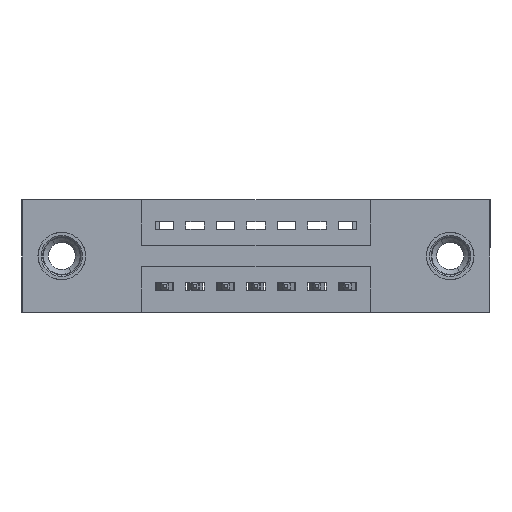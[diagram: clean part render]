
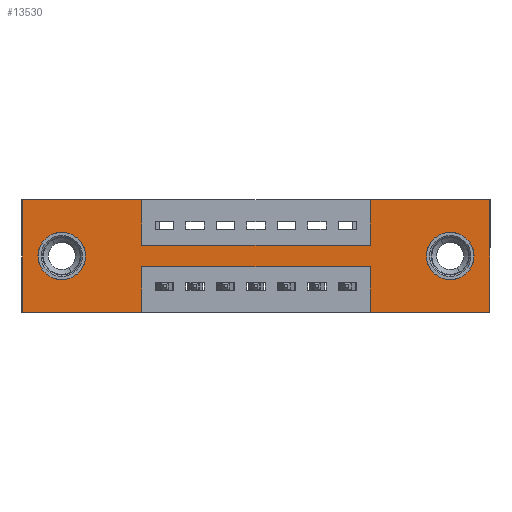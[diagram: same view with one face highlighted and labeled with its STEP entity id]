
A CAD part, front view. The second image highlights one B-rep face of the part: STEP entity #13530.
In plain terms, the highlighted planar face has unit normal (0, -1, 0).
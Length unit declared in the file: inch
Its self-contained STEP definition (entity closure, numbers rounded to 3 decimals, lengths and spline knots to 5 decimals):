
#209 = CIRCLE ( 'NONE', #303, 0.078 ) ;
#303 = AXIS2_PLACEMENT_3D ( 'NONE', #9126, #6802, #10121 ) ;
#385 = CARTESIAN_POINT ( 'NONE',  ( 0.3925, 0., -0.15 ) ) ;
#406 = VERTEX_POINT ( 'NONE', #3252 ) ;
#407 = VERTEX_POINT ( 'NONE', #1357 ) ;
#859 = DIRECTION ( 'NONE',  ( 1., 0., 0. ) ) ;
#923 = ORIENTED_EDGE ( 'NONE', *, *, #13395, .F. ) ;
#991 = EDGE_CURVE ( 'NONE', #10062, #406, #4878, .T. ) ;
#1077 = CIRCLE ( 'NONE', #7684, 0.078 ) ;
#1160 = LINE ( 'NONE', #14517, #9852 ) ;
#1196 = CARTESIAN_POINT ( 'NONE',  ( 1.1425, 0., -0.22 ) ) ;
#1280 = FACE_BOUND ( 'NONE', #7877, .T. ) ;
#1357 = CARTESIAN_POINT ( 'NONE',  ( 1.1425, 0., 0. ) ) ;
#1489 = LINE ( 'NONE', #6296, #6278 ) ;
#1538 = VERTEX_POINT ( 'NONE', #8342 ) ;
#1548 = ORIENTED_EDGE ( 'NONE', *, *, #2887, .F. ) ;
#1566 = ORIENTED_EDGE ( 'NONE', *, *, #13755, .F. ) ;
#1623 = CARTESIAN_POINT ( 'NONE',  ( 0., 0., -0.37 ) ) ;
#1640 = DIRECTION ( 'NONE',  ( 1., 0., 0. ) ) ;
#1660 = VERTEX_POINT ( 'NONE', #14369 ) ;
#1757 = CARTESIAN_POINT ( 'NONE',  ( 0.3925, 0., 0. ) ) ;
#1852 = ORIENTED_EDGE ( 'NONE', *, *, #10573, .F. ) ;
#1982 = PLANE ( 'NONE',  #3138 ) ;
#2019 = DIRECTION ( 'NONE',  ( 0., 0., 1. ) ) ;
#2030 = DIRECTION ( 'NONE',  ( 0., 0., 1. ) ) ;
#2088 = AXIS2_PLACEMENT_3D ( 'NONE', #5522, #3128, #4390 ) ;
#2141 = CARTESIAN_POINT ( 'NONE',  ( 0.13, 0., -0.107 ) ) ;
#2337 = ORIENTED_EDGE ( 'NONE', *, *, #12389, .F. ) ;
#2432 = DIRECTION ( 'NONE',  ( 0., 0., 1. ) ) ;
#2887 = EDGE_CURVE ( 'NONE', #8655, #12697, #8197, .T. ) ;
#3082 = EDGE_CURVE ( 'NONE', #406, #10062, #209, .T. ) ;
#3112 = CARTESIAN_POINT ( 'NONE',  ( 0., 0., -0.37 ) ) ;
#3128 = DIRECTION ( 'NONE',  ( 0., 1., 0. ) ) ;
#3138 = AXIS2_PLACEMENT_3D ( 'NONE', #3112, #5222, #14304 ) ;
#3252 = CARTESIAN_POINT ( 'NONE',  ( 1.405, 0., -0.107 ) ) ;
#3278 = VECTOR ( 'NONE', #859, 39.37008 ) ;
#3325 = ORIENTED_EDGE ( 'NONE', *, *, #3082, .T. ) ;
#3356 = CARTESIAN_POINT ( 'NONE',  ( 1.1425, 0., -0.37 ) ) ;
#3400 = LINE ( 'NONE', #11828, #4587 ) ;
#3623 = LINE ( 'NONE', #12787, #11231 ) ;
#3951 = DIRECTION ( 'NONE',  ( -1., 0., 0. ) ) ;
#3960 = CARTESIAN_POINT ( 'NONE',  ( 0.3925, 0., -0.37 ) ) ;
#3966 = CARTESIAN_POINT ( 'NONE',  ( 0., 0., -0.37 ) ) ;
#4141 = VECTOR ( 'NONE', #10775, 39.37008 ) ;
#4390 = DIRECTION ( 'NONE',  ( 0., 0., -1. ) ) ;
#4587 = VECTOR ( 'NONE', #3951, 39.37008 ) ;
#4605 = DIRECTION ( 'NONE',  ( 0., 0., -1. ) ) ;
#4878 = CIRCLE ( 'NONE', #2088, 0.078 ) ;
#4899 = VECTOR ( 'NONE', #10515, 39.37008 ) ;
#5222 = DIRECTION ( 'NONE',  ( 0., -1., 0. ) ) ;
#5281 = EDGE_LOOP ( 'NONE', ( #12153, #8984, #1566, #1548, #13104, #10252, #12252, #923, #10342, #2337, #1852, #14170 ) ) ;
#5294 = EDGE_CURVE ( 'NONE', #8558, #12488, #12576, .T. ) ;
#5422 = VERTEX_POINT ( 'NONE', #12933 ) ;
#5522 = CARTESIAN_POINT ( 'NONE',  ( 1.405, 0., -0.185 ) ) ;
#5589 = EDGE_CURVE ( 'NONE', #10765, #8655, #13341, .T. ) ;
#5826 = EDGE_CURVE ( 'NONE', #10266, #1660, #10973, .T. ) ;
#5904 = VECTOR ( 'NONE', #1640, 39.37008 ) ;
#6084 = CARTESIAN_POINT ( 'NONE',  ( 1.535, 0., 0. ) ) ;
#6278 = VECTOR ( 'NONE', #7489, 39.37008 ) ;
#6296 = CARTESIAN_POINT ( 'NONE',  ( 0., 0., -0.37 ) ) ;
#6699 = CARTESIAN_POINT ( 'NONE',  ( 0.13, 0., -0.263 ) ) ;
#6802 = DIRECTION ( 'NONE',  ( 0., 1., 0. ) ) ;
#7184 = CARTESIAN_POINT ( 'NONE',  ( 1.535, 0., -0.37 ) ) ;
#7489 = DIRECTION ( 'NONE',  ( -1., 0., 0. ) ) ;
#7610 = DIRECTION ( 'NONE',  ( 0., 1., 0. ) ) ;
#7684 = AXIS2_PLACEMENT_3D ( 'NONE', #10302, #12663, #2432 ) ;
#7877 = EDGE_LOOP ( 'NONE', ( #3325, #9441 ) ) ;
#8192 = VECTOR ( 'NONE', #11418, 39.37008 ) ;
#8197 = LINE ( 'NONE', #3966, #4141 ) ;
#8342 = CARTESIAN_POINT ( 'NONE',  ( 0., 0., 0. ) ) ;
#8522 = VERTEX_POINT ( 'NONE', #14728 ) ;
#8558 = VERTEX_POINT ( 'NONE', #6699 ) ;
#8655 = VERTEX_POINT ( 'NONE', #7184 ) ;
#8984 = ORIENTED_EDGE ( 'NONE', *, *, #9837, .F. ) ;
#8999 = EDGE_CURVE ( 'NONE', #407, #10765, #3623, .T. ) ;
#9126 = CARTESIAN_POINT ( 'NONE',  ( 1.405, 0., -0.185 ) ) ;
#9293 = LINE ( 'NONE', #12326, #3278 ) ;
#9441 = ORIENTED_EDGE ( 'NONE', *, *, #991, .T. ) ;
#9837 = EDGE_CURVE ( 'NONE', #14316, #8522, #3400, .T. ) ;
#9852 = VECTOR ( 'NONE', #2030, 39.37008 ) ;
#10062 = VERTEX_POINT ( 'NONE', #11763 ) ;
#10121 = DIRECTION ( 'NONE',  ( 0., 0., -1. ) ) ;
#10252 = ORIENTED_EDGE ( 'NONE', *, *, #8999, .F. ) ;
#10266 = VERTEX_POINT ( 'NONE', #1757 ) ;
#10302 = CARTESIAN_POINT ( 'NONE',  ( 0.13, 0., -0.185 ) ) ;
#10342 = ORIENTED_EDGE ( 'NONE', *, *, #5826, .F. ) ;
#10356 = CARTESIAN_POINT ( 'NONE',  ( 0.3925, 0., 0. ) ) ;
#10515 = DIRECTION ( 'NONE',  ( 0., 0., -1. ) ) ;
#10573 = EDGE_CURVE ( 'NONE', #14006, #1538, #13598, .T. ) ;
#10669 = FACE_OUTER_BOUND ( 'NONE', #5281, .T. ) ;
#10765 = VERTEX_POINT ( 'NONE', #6084 ) ;
#10775 = DIRECTION ( 'NONE',  ( -1., 0., 0. ) ) ;
#10830 = EDGE_LOOP ( 'NONE', ( #13720, #12440 ) ) ;
#10852 = LINE ( 'NONE', #385, #5904 ) ;
#10894 = LINE ( 'NONE', #3960, #4899 ) ;
#10973 = LINE ( 'NONE', #10356, #14397 ) ;
#11063 = EDGE_CURVE ( 'NONE', #8522, #5422, #10894, .T. ) ;
#11231 = VECTOR ( 'NONE', #13994, 39.37008 ) ;
#11233 = CARTESIAN_POINT ( 'NONE',  ( 0., 0., 0. ) ) ;
#11285 = DIRECTION ( 'NONE',  ( 0., 0., 1. ) ) ;
#11418 = DIRECTION ( 'NONE',  ( 0., 0., 1. ) ) ;
#11448 = VERTEX_POINT ( 'NONE', #14207 ) ;
#11537 = EDGE_CURVE ( 'NONE', #11448, #407, #1160, .T. ) ;
#11597 = CARTESIAN_POINT ( 'NONE',  ( 1.1425, 0., -0.37 ) ) ;
#11755 = FACE_BOUND ( 'NONE', #10830, .T. ) ;
#11763 = CARTESIAN_POINT ( 'NONE',  ( 1.405, 0., -0.263 ) ) ;
#11828 = CARTESIAN_POINT ( 'NONE',  ( 0.3925, 0., -0.22 ) ) ;
#11996 = VECTOR ( 'NONE', #11285, 39.37008 ) ;
#12135 = CARTESIAN_POINT ( 'NONE',  ( 0.13, 0., -0.185 ) ) ;
#12153 = ORIENTED_EDGE ( 'NONE', *, *, #11063, .F. ) ;
#12252 = ORIENTED_EDGE ( 'NONE', *, *, #11537, .F. ) ;
#12326 = CARTESIAN_POINT ( 'NONE',  ( 0., 0., 0. ) ) ;
#12389 = EDGE_CURVE ( 'NONE', #1538, #10266, #9293, .T. ) ;
#12440 = ORIENTED_EDGE ( 'NONE', *, *, #5294, .T. ) ;
#12488 = VERTEX_POINT ( 'NONE', #2141 ) ;
#12576 = CIRCLE ( 'NONE', #14717, 0.078 ) ;
#12621 = CARTESIAN_POINT ( 'NONE',  ( 1.535, 0., 0. ) ) ;
#12663 = DIRECTION ( 'NONE',  ( 0., 1., 0. ) ) ;
#12697 = VERTEX_POINT ( 'NONE', #11597 ) ;
#12772 = EDGE_CURVE ( 'NONE', #5422, #14006, #1489, .T. ) ;
#12787 = CARTESIAN_POINT ( 'NONE',  ( 0., 0., 0. ) ) ;
#12933 = CARTESIAN_POINT ( 'NONE',  ( 0.3925, 0., -0.37 ) ) ;
#13104 = ORIENTED_EDGE ( 'NONE', *, *, #5589, .F. ) ;
#13132 = DIRECTION ( 'NONE',  ( 0., 0., -1. ) ) ;
#13150 = VECTOR ( 'NONE', #4605, 39.37008 ) ;
#13341 = LINE ( 'NONE', #12621, #13150 ) ;
#13395 = EDGE_CURVE ( 'NONE', #1660, #11448, #10852, .T. ) ;
#13530 = ADVANCED_FACE ( 'NONE', ( #1280, #11755, #10669 ), #1982, .T. ) ;
#13598 = LINE ( 'NONE', #11233, #11996 ) ;
#13720 = ORIENTED_EDGE ( 'NONE', *, *, #14279, .T. ) ;
#13755 = EDGE_CURVE ( 'NONE', #12697, #14316, #14467, .T. ) ;
#13994 = DIRECTION ( 'NONE',  ( 1., 0., 0. ) ) ;
#14006 = VERTEX_POINT ( 'NONE', #1623 ) ;
#14170 = ORIENTED_EDGE ( 'NONE', *, *, #12772, .F. ) ;
#14207 = CARTESIAN_POINT ( 'NONE',  ( 1.1425, 0., -0.15 ) ) ;
#14279 = EDGE_CURVE ( 'NONE', #12488, #8558, #1077, .T. ) ;
#14304 = DIRECTION ( 'NONE',  ( 0., 0., -1. ) ) ;
#14316 = VERTEX_POINT ( 'NONE', #1196 ) ;
#14369 = CARTESIAN_POINT ( 'NONE',  ( 0.3925, 0., -0.15 ) ) ;
#14397 = VECTOR ( 'NONE', #13132, 39.37008 ) ;
#14467 = LINE ( 'NONE', #3356, #8192 ) ;
#14517 = CARTESIAN_POINT ( 'NONE',  ( 1.1425, 0., 0. ) ) ;
#14717 = AXIS2_PLACEMENT_3D ( 'NONE', #12135, #7610, #2019 ) ;
#14728 = CARTESIAN_POINT ( 'NONE',  ( 0.3925, 0., -0.22 ) ) ;
